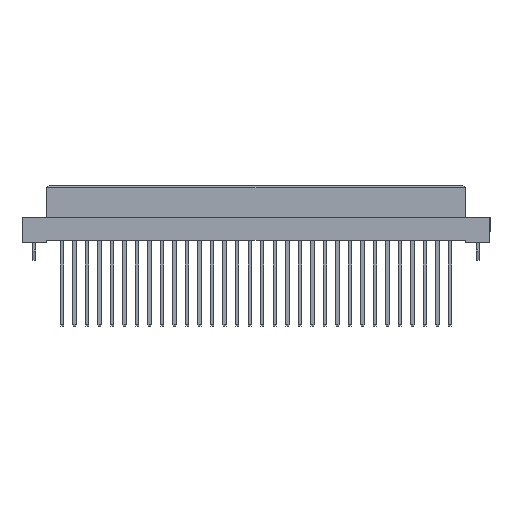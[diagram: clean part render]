
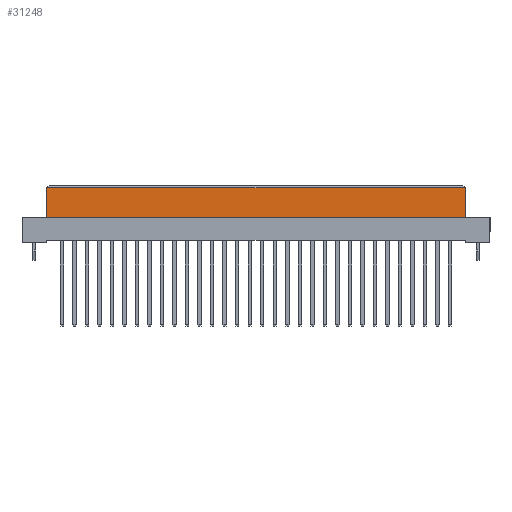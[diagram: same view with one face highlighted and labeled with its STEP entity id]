
A CAD part, top view. The second image highlights one B-rep face of the part: STEP entity #31248.
In plain terms, the highlighted planar face has unit normal (0, 0, 1).
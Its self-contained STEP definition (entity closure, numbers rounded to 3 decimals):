
#698 = LINE ( 'NONE', #8569, #22376 ) ;
#6499 = EDGE_LOOP ( 'NONE', ( #25784, #38885, #38351, #19085 ) ) ;
#7715 = VERTEX_POINT ( 'NONE', #9507 ) ;
#7975 = VECTOR ( 'NONE', #16964, 1000. ) ;
#8569 = CARTESIAN_POINT ( 'NONE',  ( 42.5, -6.4, 4.25 ) ) ;
#8771 = PLANE ( 'NONE',  #29452 ) ;
#9507 = CARTESIAN_POINT ( 'NONE',  ( 42.5, -6.4, 4.25 ) ) ;
#10839 = CARTESIAN_POINT ( 'NONE',  ( -42.5, -0.5, 4.25 ) ) ;
#11603 = VERTEX_POINT ( 'NONE', #23856 ) ;
#12351 = EDGE_CURVE ( 'NONE', #26833, #11603, #32540, .T. ) ;
#14491 = DIRECTION ( 'NONE',  ( 0., 1., 0. ) ) ;
#16637 = DIRECTION ( 'NONE',  ( 0., 1., 0. ) ) ;
#16964 = DIRECTION ( 'NONE',  ( -1., 0., 0. ) ) ;
#18316 = VERTEX_POINT ( 'NONE', #34437 ) ;
#18594 = FACE_OUTER_BOUND ( 'NONE', #6499, .T. ) ;
#19085 = ORIENTED_EDGE ( 'NONE', *, *, #33611, .T. ) ;
#20221 = EDGE_CURVE ( 'NONE', #7715, #26833, #20238, .T. ) ;
#20238 = LINE ( 'NONE', #20646, #28588 ) ;
#20646 = CARTESIAN_POINT ( 'NONE',  ( 42.5, -6.4, 4.25 ) ) ;
#21057 = DIRECTION ( 'NONE',  ( 1., 0., 0. ) ) ;
#22298 = VECTOR ( 'NONE', #16637, 1000. ) ;
#22376 = VECTOR ( 'NONE', #21057, 1000. ) ;
#22574 = CARTESIAN_POINT ( 'NONE',  ( -42.5, -6.4, 4.25 ) ) ;
#23856 = CARTESIAN_POINT ( 'NONE',  ( -42.5, -0.5, 4.25 ) ) ;
#24721 = DIRECTION ( 'NONE',  ( 0., 0., 1. ) ) ;
#25784 = ORIENTED_EDGE ( 'NONE', *, *, #20221, .T. ) ;
#26833 = VERTEX_POINT ( 'NONE', #30646 ) ;
#28588 = VECTOR ( 'NONE', #14491, 1000. ) ;
#29452 = AXIS2_PLACEMENT_3D ( 'NONE', #33955, #24721, #30482 ) ;
#30482 = DIRECTION ( 'NONE',  ( 1., 0., 0. ) ) ;
#30646 = CARTESIAN_POINT ( 'NONE',  ( 42.5, -0.5, 4.25 ) ) ;
#31248 = ADVANCED_FACE ( 'NONE', ( #18594 ), #8771, .T. ) ;
#31860 = EDGE_CURVE ( 'NONE', #18316, #11603, #35669, .T. ) ;
#32540 = LINE ( 'NONE', #10839, #7975 ) ;
#33611 = EDGE_CURVE ( 'NONE', #18316, #7715, #698, .T. ) ;
#33955 = CARTESIAN_POINT ( 'NONE',  ( 42.5, -6.4, 4.25 ) ) ;
#34437 = CARTESIAN_POINT ( 'NONE',  ( -42.5, -6.4, 4.25 ) ) ;
#35669 = LINE ( 'NONE', #22574, #22298 ) ;
#38351 = ORIENTED_EDGE ( 'NONE', *, *, #31860, .F. ) ;
#38885 = ORIENTED_EDGE ( 'NONE', *, *, #12351, .T. ) ;
